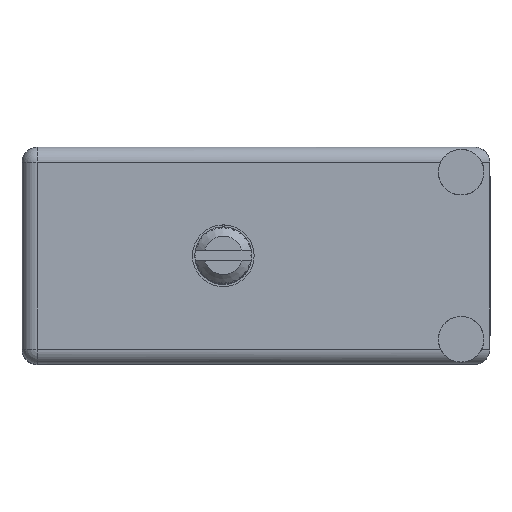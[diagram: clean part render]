
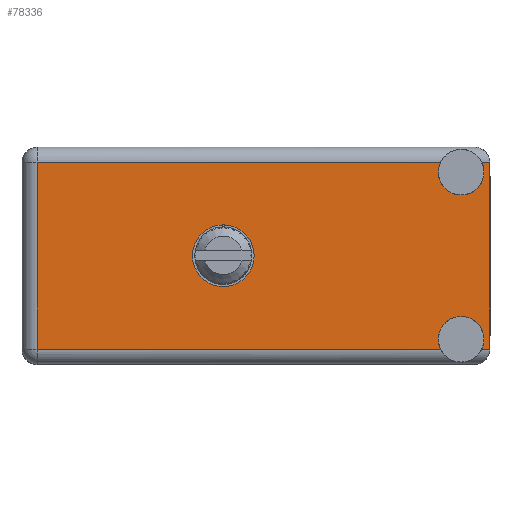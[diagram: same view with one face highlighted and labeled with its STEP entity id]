
A CAD part, top view. The second image highlights one B-rep face of the part: STEP entity #78336.
In plain terms, the highlighted face is planar.
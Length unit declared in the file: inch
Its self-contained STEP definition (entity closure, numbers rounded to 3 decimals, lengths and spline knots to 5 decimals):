
#1460 = EDGE_CURVE ( 'NONE', #194031, #31670, #27960, .T. ) ;
#1760 = ORIENTED_EDGE ( 'NONE', *, *, #121043, .F. ) ;
#3131 = ORIENTED_EDGE ( 'NONE', *, *, #131510, .F. ) ;
#6331 = CARTESIAN_POINT ( 'NONE',  ( 0., 0.806, 0. ) ) ;
#6907 = VECTOR ( 'NONE', #44066, 39.37008 ) ;
#7291 = CIRCLE ( 'NONE', #23406, 0.075 ) ;
#13824 = DIRECTION ( 'NONE',  ( 0., 0., 1. ) ) ;
#14168 = AXIS2_PLACEMENT_3D ( 'NONE', #6331, #114267, #82951 ) ;
#14593 = VECTOR ( 'NONE', #150619, 39.37008 ) ;
#18614 = ORIENTED_EDGE ( 'NONE', *, *, #192164, .T. ) ;
#21023 = CARTESIAN_POINT ( 'NONE',  ( 0.7825, 0.806, -0.275 ) ) ;
#22497 = DIRECTION ( 'NONE',  ( 0., 1., 0. ) ) ;
#23325 = EDGE_CURVE ( 'NONE', #83401, #33917, #136659, .T. ) ;
#23406 = AXIS2_PLACEMENT_3D ( 'NONE', #61000, #122546, #168954 ) ;
#25492 = FACE_BOUND ( 'NONE', #30100, .T. ) ;
#27774 = LINE ( 'NONE', #28767, #157820 ) ;
#27960 = LINE ( 'NONE', #74298, #6907 ) ;
#28767 = CARTESIAN_POINT ( 'NONE',  ( -0.6125, 0.806, -0.3575 ) ) ;
#30100 = EDGE_LOOP ( 'NONE', ( #93189, #172428 ) ) ;
#31670 = VERTEX_POINT ( 'NONE', #197972 ) ;
#32050 = EDGE_CURVE ( 'NONE', #70602, #92019, #76454, .T. ) ;
#33917 = VERTEX_POINT ( 'NONE', #76413 ) ;
#37039 = DIRECTION ( 'NONE',  ( 1., 0., 0. ) ) ;
#38593 = PLANE ( 'NONE',  #151888 ) ;
#38715 = DIRECTION ( 'NONE',  ( 0., 0., 1. ) ) ;
#39111 = DIRECTION ( 'NONE',  ( 0., 0., 1. ) ) ;
#40267 = VERTEX_POINT ( 'NONE', #83093 ) ;
#40989 = VERTEX_POINT ( 'NONE', #90974 ) ;
#41506 = CARTESIAN_POINT ( 'NONE',  ( 0., 0.806, 0. ) ) ;
#41517 = EDGE_CURVE ( 'NONE', #155973, #183310, #7291, .T. ) ;
#43093 = CARTESIAN_POINT ( 'NONE',  ( 0.7825, 0.806, -0.275 ) ) ;
#44066 = DIRECTION ( 'NONE',  ( 0., 0., 1. ) ) ;
#53236 = CARTESIAN_POINT ( 'NONE',  ( 0.85009, 0.806, -0.3075 ) ) ;
#53526 = CIRCLE ( 'NONE', #114750, 0.1015 ) ;
#53743 = CARTESIAN_POINT ( 'NONE',  ( -0.6625, 0.806, -0.3575 ) ) ;
#57652 = DIRECTION ( 'NONE',  ( 0., 0., 1. ) ) ;
#58565 = CARTESIAN_POINT ( 'NONE',  ( -0.6625, 0.806, -0.3075 ) ) ;
#58794 = VERTEX_POINT ( 'NONE', #116234 ) ;
#61000 = CARTESIAN_POINT ( 'NONE',  ( 0.7825, 0.806, 0.275 ) ) ;
#70602 = VERTEX_POINT ( 'NONE', #80210 ) ;
#71288 = ORIENTED_EDGE ( 'NONE', *, *, #171815, .T. ) ;
#73284 = CARTESIAN_POINT ( 'NONE',  ( 0.71491, 0.806, 0.3075 ) ) ;
#73741 = DIRECTION ( 'NONE',  ( 0., 1., 0. ) ) ;
#74298 = CARTESIAN_POINT ( 'NONE',  ( 0.8765, 0.806, 0.3575 ) ) ;
#76413 = CARTESIAN_POINT ( 'NONE',  ( -0.6125, 0.806, -0.3075 ) ) ;
#76454 = CIRCLE ( 'NONE', #157109, 0.075 ) ;
#77455 = AXIS2_PLACEMENT_3D ( 'NONE', #164805, #180011, #38715 ) ;
#78164 = AXIS2_PLACEMENT_3D ( 'NONE', #43093, #138866, #13824 ) ;
#78336 = ADVANCED_FACE ( 'NONE', ( #25492, #164674 ), #38593, .T. ) ;
#80210 = CARTESIAN_POINT ( 'NONE',  ( 0.7825, 0.806, -0.2 ) ) ;
#82951 = DIRECTION ( 'NONE',  ( 0., 0., 1. ) ) ;
#83093 = CARTESIAN_POINT ( 'NONE',  ( 0., 0.806, 0.1015 ) ) ;
#83401 = VERTEX_POINT ( 'NONE', #106819 ) ;
#89085 = CARTESIAN_POINT ( 'NONE',  ( 0.8765, 0.806, 0.3075 ) ) ;
#90974 = CARTESIAN_POINT ( 'NONE',  ( 0.85009, 0.806, 0.3075 ) ) ;
#92019 = VERTEX_POINT ( 'NONE', #53236 ) ;
#92226 = CARTESIAN_POINT ( 'NONE',  ( -0.6625, 0.806, -0.3075 ) ) ;
#93189 = ORIENTED_EDGE ( 'NONE', *, *, #167450, .F. ) ;
#95591 = LINE ( 'NONE', #175278, #165810 ) ;
#100066 = ORIENTED_EDGE ( 'NONE', *, *, #23325, .T. ) ;
#106819 = CARTESIAN_POINT ( 'NONE',  ( 0.71491, 0.806, -0.3075 ) ) ;
#108172 = VECTOR ( 'NONE', #121134, 39.37008 ) ;
#114267 = DIRECTION ( 'NONE',  ( 0., 1., 0. ) ) ;
#114750 = AXIS2_PLACEMENT_3D ( 'NONE', #41506, #73741, #57652 ) ;
#116234 = CARTESIAN_POINT ( 'NONE',  ( -0.6125, 0.806, 0.3075 ) ) ;
#120125 = LINE ( 'NONE', #58565, #108172 ) ;
#120809 = ORIENTED_EDGE ( 'NONE', *, *, #1460, .F. ) ;
#121043 = EDGE_CURVE ( 'NONE', #40989, #155973, #135981, .T. ) ;
#121134 = DIRECTION ( 'NONE',  ( -1., 0., 0. ) ) ;
#122546 = DIRECTION ( 'NONE',  ( 0., 1., 0. ) ) ;
#122563 = DIRECTION ( 'NONE',  ( 0., 0., 1. ) ) ;
#130725 = CARTESIAN_POINT ( 'NONE',  ( 0., 0.806, -0.1015 ) ) ;
#131510 = EDGE_CURVE ( 'NONE', #83401, #70602, #152354, .T. ) ;
#135981 = CIRCLE ( 'NONE', #77455, 0.075 ) ;
#136659 = LINE ( 'NONE', #92226, #192886 ) ;
#138866 = DIRECTION ( 'NONE',  ( 0., 1., 0. ) ) ;
#142284 = ORIENTED_EDGE ( 'NONE', *, *, #32050, .F. ) ;
#142308 = VERTEX_POINT ( 'NONE', #130725 ) ;
#142378 = CARTESIAN_POINT ( 'NONE',  ( 0.8765, 0.806, -0.3075 ) ) ;
#145179 = CARTESIAN_POINT ( 'NONE',  ( 0.7825, 0.806, 0.2 ) ) ;
#147874 = EDGE_CURVE ( 'NONE', #194031, #92019, #120125, .T. ) ;
#149369 = CIRCLE ( 'NONE', #14168, 0.1015 ) ;
#149418 = ORIENTED_EDGE ( 'NONE', *, *, #147874, .T. ) ;
#150619 = DIRECTION ( 'NONE',  ( 1., 0., 0. ) ) ;
#151888 = AXIS2_PLACEMENT_3D ( 'NONE', #53743, #22497, #179881 ) ;
#152354 = CIRCLE ( 'NONE', #78164, 0.075 ) ;
#155973 = VERTEX_POINT ( 'NONE', #145179 ) ;
#157109 = AXIS2_PLACEMENT_3D ( 'NONE', #21023, #191535, #39111 ) ;
#157820 = VECTOR ( 'NONE', #122563, 39.37008 ) ;
#159349 = EDGE_CURVE ( 'NONE', #142308, #40267, #53526, .T. ) ;
#164674 = FACE_OUTER_BOUND ( 'NONE', #190874, .T. ) ;
#164805 = CARTESIAN_POINT ( 'NONE',  ( 0.7825, 0.806, 0.275 ) ) ;
#165810 = VECTOR ( 'NONE', #37039, 39.37008 ) ;
#166936 = DIRECTION ( 'NONE',  ( -1., 0., 0. ) ) ;
#167450 = EDGE_CURVE ( 'NONE', #40267, #142308, #149369, .T. ) ;
#167961 = ORIENTED_EDGE ( 'NONE', *, *, #174966, .T. ) ;
#168954 = DIRECTION ( 'NONE',  ( 0., 0., 1. ) ) ;
#171815 = EDGE_CURVE ( 'NONE', #40989, #31670, #95591, .T. ) ;
#172428 = ORIENTED_EDGE ( 'NONE', *, *, #159349, .F. ) ;
#174966 = EDGE_CURVE ( 'NONE', #58794, #183310, #180960, .T. ) ;
#175278 = CARTESIAN_POINT ( 'NONE',  ( 0.8765, 0.806, 0.3075 ) ) ;
#177284 = ORIENTED_EDGE ( 'NONE', *, *, #41517, .F. ) ;
#179881 = DIRECTION ( 'NONE',  ( -1., 0., 0. ) ) ;
#180011 = DIRECTION ( 'NONE',  ( 0., 1., 0. ) ) ;
#180960 = LINE ( 'NONE', #89085, #14593 ) ;
#183310 = VERTEX_POINT ( 'NONE', #73284 ) ;
#190874 = EDGE_LOOP ( 'NONE', ( #167961, #177284, #1760, #71288, #120809, #149418, #142284, #3131, #100066, #18614 ) ) ;
#191535 = DIRECTION ( 'NONE',  ( 0., 1., 0. ) ) ;
#192164 = EDGE_CURVE ( 'NONE', #33917, #58794, #27774, .T. ) ;
#192886 = VECTOR ( 'NONE', #166936, 39.37008 ) ;
#194031 = VERTEX_POINT ( 'NONE', #142378 ) ;
#197972 = CARTESIAN_POINT ( 'NONE',  ( 0.8765, 0.806, 0.3075 ) ) ;
